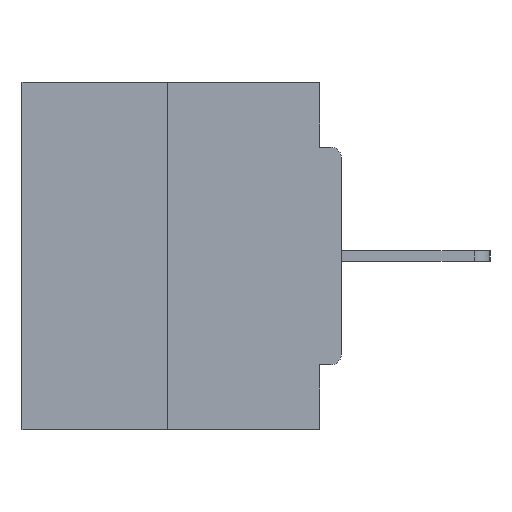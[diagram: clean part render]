
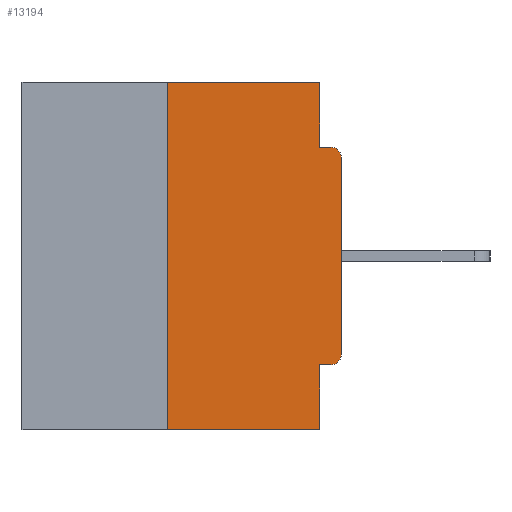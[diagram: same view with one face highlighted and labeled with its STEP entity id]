
A CAD part, left-side view. The second image highlights one B-rep face of the part: STEP entity #13194.
In plain terms, the highlighted planar face has unit normal (-1, 0, 0).
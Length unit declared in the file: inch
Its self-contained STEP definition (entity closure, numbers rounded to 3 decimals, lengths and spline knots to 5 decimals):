
#91 = DIRECTION ( 'NONE',  ( 0., -1., 0. ) ) ;
#640 = CARTESIAN_POINT ( 'NONE',  ( 0., 0., -0.1085 ) ) ;
#772 = VERTEX_POINT ( 'NONE', #3855 ) ;
#1077 = LINE ( 'NONE', #8656, #25104 ) ;
#1097 = PLANE ( 'NONE',  #12773 ) ;
#1247 = CARTESIAN_POINT ( 'NONE',  ( 0., 0.46, 0. ) ) ;
#2559 = ORIENTED_EDGE ( 'NONE', *, *, #10914, .F. ) ;
#2576 = CARTESIAN_POINT ( 'NONE',  ( 0., 0., -0.4065 ) ) ;
#2905 = CARTESIAN_POINT ( 'NONE',  ( 0., 0.031, -0.0935 ) ) ;
#3545 = DIRECTION ( 'NONE',  ( 0., 0., -1. ) ) ;
#3825 = LINE ( 'NONE', #11535, #5208 ) ;
#3855 = CARTESIAN_POINT ( 'NONE',  ( 0., 0., -0.3915 ) ) ;
#4944 = AXIS2_PLACEMENT_3D ( 'NONE', #13664, #21265, #3545 ) ;
#5087 = CARTESIAN_POINT ( 'NONE',  ( 0., 0.46, -0.5 ) ) ;
#5208 = VECTOR ( 'NONE', #13633, 39.37008 ) ;
#5374 = DIRECTION ( 'NONE',  ( 0., 0., 1. ) ) ;
#5778 = DIRECTION ( 'NONE',  ( 0., 0., -1. ) ) ;
#6095 = FACE_OUTER_BOUND ( 'NONE', #12366, .T. ) ;
#6105 = VECTOR ( 'NONE', #5374, 39.37008 ) ;
#6135 = DIRECTION ( 'NONE',  ( -1., 0., 0. ) ) ;
#6226 = VECTOR ( 'NONE', #10912, 39.37008 ) ;
#7425 = ORIENTED_EDGE ( 'NONE', *, *, #28924, .F. ) ;
#7771 = CARTESIAN_POINT ( 'NONE',  ( 0., 0.46, 0. ) ) ;
#8135 = ORIENTED_EDGE ( 'NONE', *, *, #25595, .F. ) ;
#8374 = DIRECTION ( 'NONE',  ( 0., -1., 0. ) ) ;
#8473 = VERTEX_POINT ( 'NONE', #25991 ) ;
#8656 = CARTESIAN_POINT ( 'NONE',  ( 0., 0.031, -0.5 ) ) ;
#8677 = VERTEX_POINT ( 'NONE', #640 ) ;
#8874 = DIRECTION ( 'NONE',  ( 0., 0., -1. ) ) ;
#9776 = LINE ( 'NONE', #5087, #20498 ) ;
#10288 = VERTEX_POINT ( 'NONE', #20784 ) ;
#10349 = DIRECTION ( 'NONE',  ( 0., 0., -1. ) ) ;
#10751 = LINE ( 'NONE', #20580, #6226 ) ;
#10912 = DIRECTION ( 'NONE',  ( 0., 0., 1. ) ) ;
#10914 = EDGE_CURVE ( 'NONE', #17323, #8473, #3825, .T. ) ;
#11271 = CARTESIAN_POINT ( 'NONE',  ( 0., 0.015, -0.1085 ) ) ;
#11535 = CARTESIAN_POINT ( 'NONE',  ( 0., 0., -0.0935 ) ) ;
#12285 = LINE ( 'NONE', #22457, #6105 ) ;
#12366 = EDGE_LOOP ( 'NONE', ( #7425, #31224, #16182, #8135, #27396, #25282, #29920, #14433, #2559, #18580 ) ) ;
#12433 = VERTEX_POINT ( 'NONE', #20243 ) ;
#12773 = AXIS2_PLACEMENT_3D ( 'NONE', #7771, #23192, #19990 ) ;
#13194 = ADVANCED_FACE ( 'NONE', ( #6095 ), #1097, .F. ) ;
#13233 = CIRCLE ( 'NONE', #19935, 0.015 ) ;
#13383 = VECTOR ( 'NONE', #8374, 39.37008 ) ;
#13633 = DIRECTION ( 'NONE',  ( 0., -1., 0. ) ) ;
#13642 = CARTESIAN_POINT ( 'NONE',  ( 0., 0.25, 0. ) ) ;
#13664 = CARTESIAN_POINT ( 'NONE',  ( 0., 0.015, -0.3915 ) ) ;
#14282 = EDGE_CURVE ( 'NONE', #12433, #15645, #31177, .T. ) ;
#14433 = ORIENTED_EDGE ( 'NONE', *, *, #20803, .T. ) ;
#15032 = EDGE_CURVE ( 'NONE', #772, #8677, #10751, .T. ) ;
#15274 = VECTOR ( 'NONE', #10349, 39.37008 ) ;
#15645 = VERTEX_POINT ( 'NONE', #23756 ) ;
#16182 = ORIENTED_EDGE ( 'NONE', *, *, #21715, .T. ) ;
#17323 = VERTEX_POINT ( 'NONE', #2905 ) ;
#18580 = ORIENTED_EDGE ( 'NONE', *, *, #25154, .F. ) ;
#19522 = EDGE_CURVE ( 'NONE', #12433, #772, #22468, .T. ) ;
#19935 = AXIS2_PLACEMENT_3D ( 'NONE', #11271, #6135, #8874 ) ;
#19990 = DIRECTION ( 'NONE',  ( 0., 0., -1. ) ) ;
#20243 = CARTESIAN_POINT ( 'NONE',  ( 0., 0.015, -0.4065 ) ) ;
#20498 = VECTOR ( 'NONE', #91, 39.37008 ) ;
#20522 = VERTEX_POINT ( 'NONE', #24215 ) ;
#20580 = CARTESIAN_POINT ( 'NONE',  ( 0., 0., 0. ) ) ;
#20594 = CARTESIAN_POINT ( 'NONE',  ( 0., 0.031, -0.5 ) ) ;
#20784 = CARTESIAN_POINT ( 'NONE',  ( 0., 0.25, -0.5 ) ) ;
#20803 = EDGE_CURVE ( 'NONE', #8677, #8473, #13233, .T. ) ;
#21265 = DIRECTION ( 'NONE',  ( -1., 0., 0. ) ) ;
#21715 = EDGE_CURVE ( 'NONE', #10288, #22774, #9776, .T. ) ;
#22457 = CARTESIAN_POINT ( 'NONE',  ( 0., 0.25, 0. ) ) ;
#22468 = CIRCLE ( 'NONE', #4944, 0.015 ) ;
#22774 = VERTEX_POINT ( 'NONE', #20594 ) ;
#23192 = DIRECTION ( 'NONE',  ( 1., 0., 0. ) ) ;
#23756 = CARTESIAN_POINT ( 'NONE',  ( 0., 0.031, -0.4065 ) ) ;
#24184 = VECTOR ( 'NONE', #24498, 39.37008 ) ;
#24215 = CARTESIAN_POINT ( 'NONE',  ( 0., 0.031, 0. ) ) ;
#24498 = DIRECTION ( 'NONE',  ( 0., 1., 0. ) ) ;
#25104 = VECTOR ( 'NONE', #5778, 39.37008 ) ;
#25154 = EDGE_CURVE ( 'NONE', #20522, #17323, #27105, .T. ) ;
#25282 = ORIENTED_EDGE ( 'NONE', *, *, #19522, .T. ) ;
#25595 = EDGE_CURVE ( 'NONE', #15645, #22774, #1077, .T. ) ;
#25991 = CARTESIAN_POINT ( 'NONE',  ( 0., 0.015, -0.0935 ) ) ;
#26111 = VERTEX_POINT ( 'NONE', #13642 ) ;
#27105 = LINE ( 'NONE', #29545, #15274 ) ;
#27396 = ORIENTED_EDGE ( 'NONE', *, *, #14282, .F. ) ;
#28924 = EDGE_CURVE ( 'NONE', #26111, #20522, #30491, .T. ) ;
#29545 = CARTESIAN_POINT ( 'NONE',  ( 0., 0.031, 0. ) ) ;
#29920 = ORIENTED_EDGE ( 'NONE', *, *, #15032, .T. ) ;
#30491 = LINE ( 'NONE', #1247, #13383 ) ;
#30705 = EDGE_CURVE ( 'NONE', #10288, #26111, #12285, .T. ) ;
#31177 = LINE ( 'NONE', #2576, #24184 ) ;
#31224 = ORIENTED_EDGE ( 'NONE', *, *, #30705, .F. ) ;
